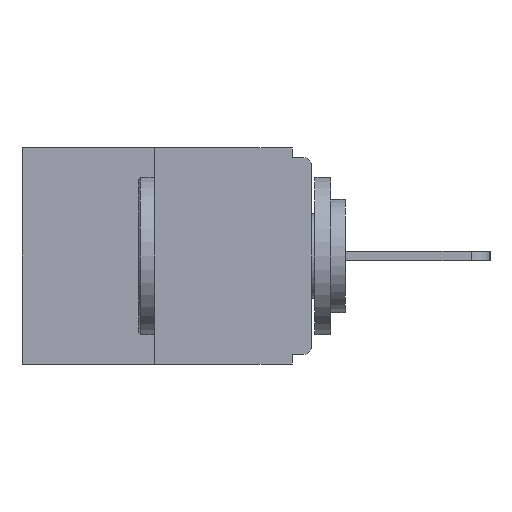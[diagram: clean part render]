
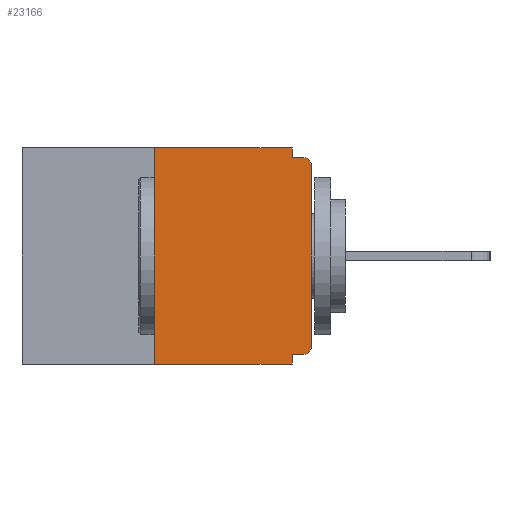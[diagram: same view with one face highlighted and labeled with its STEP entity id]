
A CAD part, left-side view. The second image highlights one B-rep face of the part: STEP entity #23166.
In plain terms, the highlighted planar face has unit normal (-1, 0, 0).
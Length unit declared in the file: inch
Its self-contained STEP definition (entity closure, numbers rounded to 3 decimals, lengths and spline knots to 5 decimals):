
#164 = ORIENTED_EDGE ( 'NONE', *, *, #2423, .F. ) ;
#978 = CARTESIAN_POINT ( 'NONE',  ( 0., 0.031, -0.015 ) ) ;
#1064 = EDGE_CURVE ( 'NONE', #8047, #24245, #12901, .T. ) ;
#1754 = CARTESIAN_POINT ( 'NONE',  ( 0., 0.25, -0.343 ) ) ;
#2423 = EDGE_CURVE ( 'NONE', #8047, #9373, #13110, .T. ) ;
#2773 = EDGE_CURVE ( 'NONE', #12004, #23939, #14889, .T. ) ;
#2951 = CIRCLE ( 'NONE', #19407, 0.015 ) ;
#3346 = ORIENTED_EDGE ( 'NONE', *, *, #22650, .F. ) ;
#3743 = CIRCLE ( 'NONE', #21868, 0.015 ) ;
#3852 = DIRECTION ( 'NONE',  ( 0., -1., 0. ) ) ;
#4166 = CARTESIAN_POINT ( 'NONE',  ( 0., 0.015, -0.015 ) ) ;
#4755 = CARTESIAN_POINT ( 'NONE',  ( 0., 0.46, 0. ) ) ;
#4976 = VECTOR ( 'NONE', #3852, 39.37008 ) ;
#5466 = CARTESIAN_POINT ( 'NONE',  ( 0., 0., -0.328 ) ) ;
#6028 = CARTESIAN_POINT ( 'NONE',  ( 0., 0.031, 0. ) ) ;
#6757 = DIRECTION ( 'NONE',  ( 0., 0., -1. ) ) ;
#6830 = CARTESIAN_POINT ( 'NONE',  ( 0., 0.015, -0.03 ) ) ;
#7212 = VECTOR ( 'NONE', #18761, 39.37008 ) ;
#7309 = DIRECTION ( 'NONE',  ( 0., -1., 0. ) ) ;
#7375 = ORIENTED_EDGE ( 'NONE', *, *, #2773, .F. ) ;
#7432 = CARTESIAN_POINT ( 'NONE',  ( 0., 0.031, -0.328 ) ) ;
#8047 = VERTEX_POINT ( 'NONE', #1754 ) ;
#8060 = VERTEX_POINT ( 'NONE', #11532 ) ;
#8082 = EDGE_CURVE ( 'NONE', #8060, #10843, #20526, .T. ) ;
#8145 = DIRECTION ( 'NONE',  ( 0., 0., -1. ) ) ;
#8798 = DIRECTION ( 'NONE',  ( 0., 0., -1. ) ) ;
#8956 = AXIS2_PLACEMENT_3D ( 'NONE', #4755, #18241, #6757 ) ;
#9373 = VERTEX_POINT ( 'NONE', #9896 ) ;
#9752 = VECTOR ( 'NONE', #7309, 39.37008 ) ;
#9787 = DIRECTION ( 'NONE',  ( 0., 0., 1. ) ) ;
#9896 = CARTESIAN_POINT ( 'NONE',  ( 0., 0.25, 0. ) ) ;
#10048 = DIRECTION ( 'NONE',  ( -1., 0., 0. ) ) ;
#10175 = FACE_OUTER_BOUND ( 'NONE', #15681, .T. ) ;
#10763 = LINE ( 'NONE', #6028, #11956 ) ;
#10843 = VERTEX_POINT ( 'NONE', #20087 ) ;
#11006 = VECTOR ( 'NONE', #9787, 39.37008 ) ;
#11532 = CARTESIAN_POINT ( 'NONE',  ( 0., 0., -0.313 ) ) ;
#11601 = VERTEX_POINT ( 'NONE', #978 ) ;
#11956 = VECTOR ( 'NONE', #17545, 39.37008 ) ;
#12004 = VERTEX_POINT ( 'NONE', #23479 ) ;
#12901 = LINE ( 'NONE', #18710, #7212 ) ;
#13110 = LINE ( 'NONE', #22734, #13701 ) ;
#13619 = VECTOR ( 'NONE', #8145, 39.37008 ) ;
#13678 = VECTOR ( 'NONE', #25052, 39.37008 ) ;
#13701 = VECTOR ( 'NONE', #16212, 39.37008 ) ;
#14098 = CARTESIAN_POINT ( 'NONE',  ( 0., 0.031, -0.343 ) ) ;
#14427 = CARTESIAN_POINT ( 'NONE',  ( 0., 0.031, 0. ) ) ;
#14781 = LINE ( 'NONE', #20698, #9752 ) ;
#14889 = LINE ( 'NONE', #5466, #13678 ) ;
#15222 = LINE ( 'NONE', #17359, #4976 ) ;
#15681 = EDGE_LOOP ( 'NONE', ( #20245, #164, #16319, #21459, #7375, #17544, #22642, #18156, #3346, #23848 ) ) ;
#16212 = DIRECTION ( 'NONE',  ( 0., 0., 1. ) ) ;
#16282 = PLANE ( 'NONE',  #8956 ) ;
#16319 = ORIENTED_EDGE ( 'NONE', *, *, #1064, .T. ) ;
#17359 = CARTESIAN_POINT ( 'NONE',  ( 0., 0.46, 0. ) ) ;
#17515 = EDGE_CURVE ( 'NONE', #10843, #24893, #2951, .T. ) ;
#17544 = ORIENTED_EDGE ( 'NONE', *, *, #20075, .T. ) ;
#17545 = DIRECTION ( 'NONE',  ( 0., 0., -1. ) ) ;
#18156 = ORIENTED_EDGE ( 'NONE', *, *, #17515, .T. ) ;
#18241 = DIRECTION ( 'NONE',  ( 1., 0., 0. ) ) ;
#18710 = CARTESIAN_POINT ( 'NONE',  ( 0., 0.46, -0.343 ) ) ;
#18761 = DIRECTION ( 'NONE',  ( 0., -1., 0. ) ) ;
#19407 = AXIS2_PLACEMENT_3D ( 'NONE', #6830, #20237, #8798 ) ;
#19593 = CARTESIAN_POINT ( 'NONE',  ( 0., 0.031, -0.343 ) ) ;
#19971 = EDGE_CURVE ( 'NONE', #9373, #22471, #15222, .T. ) ;
#20075 = EDGE_CURVE ( 'NONE', #12004, #8060, #3743, .T. ) ;
#20087 = CARTESIAN_POINT ( 'NONE',  ( 0., 0., -0.03 ) ) ;
#20237 = DIRECTION ( 'NONE',  ( -1., 0., 0. ) ) ;
#20245 = ORIENTED_EDGE ( 'NONE', *, *, #19971, .F. ) ;
#20526 = LINE ( 'NONE', #21216, #11006 ) ;
#20698 = CARTESIAN_POINT ( 'NONE',  ( 0., 0., -0.015 ) ) ;
#21216 = CARTESIAN_POINT ( 'NONE',  ( 0., 0., 0. ) ) ;
#21459 = ORIENTED_EDGE ( 'NONE', *, *, #24889, .F. ) ;
#21480 = CARTESIAN_POINT ( 'NONE',  ( 0., 0.015, -0.313 ) ) ;
#21868 = AXIS2_PLACEMENT_3D ( 'NONE', #21480, #10048, #23379 ) ;
#22471 = VERTEX_POINT ( 'NONE', #14427 ) ;
#22642 = ORIENTED_EDGE ( 'NONE', *, *, #8082, .T. ) ;
#22650 = EDGE_CURVE ( 'NONE', #11601, #24893, #14781, .T. ) ;
#22734 = CARTESIAN_POINT ( 'NONE',  ( 0., 0.25, 0. ) ) ;
#23166 = ADVANCED_FACE ( 'NONE', ( #10175 ), #16282, .F. ) ;
#23379 = DIRECTION ( 'NONE',  ( 0., 0., -1. ) ) ;
#23479 = CARTESIAN_POINT ( 'NONE',  ( 0., 0.015, -0.328 ) ) ;
#23611 = EDGE_CURVE ( 'NONE', #22471, #11601, #10763, .T. ) ;
#23848 = ORIENTED_EDGE ( 'NONE', *, *, #23611, .F. ) ;
#23939 = VERTEX_POINT ( 'NONE', #7432 ) ;
#24245 = VERTEX_POINT ( 'NONE', #14098 ) ;
#24889 = EDGE_CURVE ( 'NONE', #23939, #24245, #25025, .T. ) ;
#24893 = VERTEX_POINT ( 'NONE', #4166 ) ;
#25025 = LINE ( 'NONE', #19593, #13619 ) ;
#25052 = DIRECTION ( 'NONE',  ( 0., 1., 0. ) ) ;
